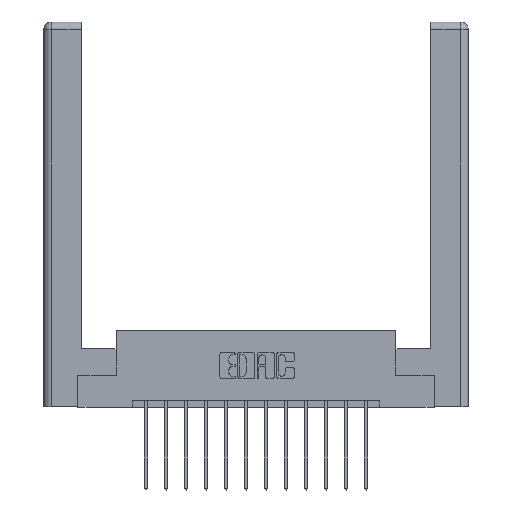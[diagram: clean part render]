
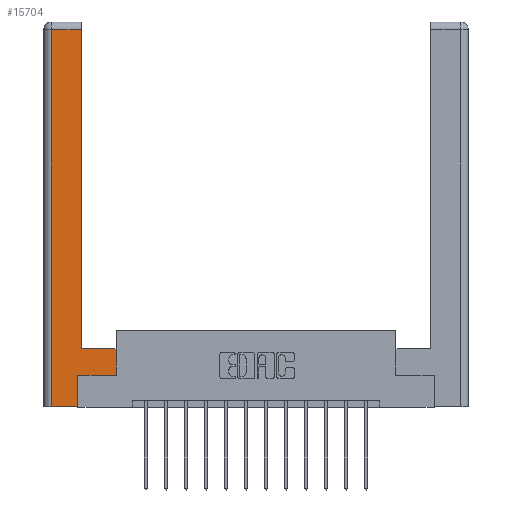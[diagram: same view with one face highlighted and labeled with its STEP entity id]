
A CAD part, top view. The second image highlights one B-rep face of the part: STEP entity #15704.
In plain terms, the highlighted planar face has unit normal (0, 0, 1).
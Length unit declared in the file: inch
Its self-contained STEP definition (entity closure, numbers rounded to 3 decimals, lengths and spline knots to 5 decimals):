
#34 = LINE ( 'NONE', #11506, #3421 ) ;
#152 = EDGE_CURVE ( 'NONE', #5660, #15445, #3620, .T. ) ;
#252 = VERTEX_POINT ( 'NONE', #13423 ) ;
#320 = CARTESIAN_POINT ( 'NONE',  ( 0.265, 0.245, 0. ) ) ;
#393 = CARTESIAN_POINT ( 'NONE',  ( 0.265, 0., 0. ) ) ;
#1141 = FACE_OUTER_BOUND ( 'NONE', #15610, .T. ) ;
#2104 = LINE ( 'NONE', #10669, #11494 ) ;
#2165 = LINE ( 'NONE', #12071, #10993 ) ;
#2635 = VERTEX_POINT ( 'NONE', #12365 ) ;
#2739 = CARTESIAN_POINT ( 'NONE',  ( 0.565, 0.45, 0. ) ) ;
#3310 = DIRECTION ( 'NONE',  ( -1., 0., 0. ) ) ;
#3421 = VECTOR ( 'NONE', #7857, 39.37008 ) ;
#3486 = ORIENTED_EDGE ( 'NONE', *, *, #6939, .T. ) ;
#3620 = LINE ( 'NONE', #11770, #6904 ) ;
#3713 = CARTESIAN_POINT ( 'NONE',  ( 0.0615, 0., 0. ) ) ;
#3792 = ORIENTED_EDGE ( 'NONE', *, *, #14293, .T. ) ;
#3979 = LINE ( 'NONE', #14319, #15554 ) ;
#4308 = ORIENTED_EDGE ( 'NONE', *, *, #7170, .T. ) ;
#4448 = LINE ( 'NONE', #320, #5607 ) ;
#4480 = DIRECTION ( 'NONE',  ( -1., 0., 0. ) ) ;
#4571 = DIRECTION ( 'NONE',  ( 0., 1., 0. ) ) ;
#4984 = CARTESIAN_POINT ( 'NONE',  ( 0.265, 0.245, 0. ) ) ;
#5185 = ORIENTED_EDGE ( 'NONE', *, *, #152, .T. ) ;
#5607 = VECTOR ( 'NONE', #4571, 39.37008 ) ;
#5660 = VERTEX_POINT ( 'NONE', #4984 ) ;
#6153 = VECTOR ( 'NONE', #13874, 39.37008 ) ;
#6904 = VECTOR ( 'NONE', #9497, 39.37008 ) ;
#6939 = EDGE_CURVE ( 'NONE', #7324, #252, #2165, .T. ) ;
#7100 = ORIENTED_EDGE ( 'NONE', *, *, #7383, .T. ) ;
#7170 = EDGE_CURVE ( 'NONE', #2635, #5660, #4448, .T. ) ;
#7324 = VERTEX_POINT ( 'NONE', #9825 ) ;
#7352 = VECTOR ( 'NONE', #12572, 39.37008 ) ;
#7383 = EDGE_CURVE ( 'NONE', #15445, #14016, #15800, .T. ) ;
#7563 = VERTEX_POINT ( 'NONE', #3713 ) ;
#7857 = DIRECTION ( 'NONE',  ( 0., -1., 0. ) ) ;
#8174 = EDGE_CURVE ( 'NONE', #7563, #2635, #12693, .T. ) ;
#8205 = CARTESIAN_POINT ( 'NONE',  ( 0.0615, 2.94, 0. ) ) ;
#8417 = DIRECTION ( 'NONE',  ( 0., 0., -1. ) ) ;
#9130 = EDGE_CURVE ( 'NONE', #14016, #7324, #3979, .T. ) ;
#9189 = EDGE_CURVE ( 'NONE', #252, #15687, #2104, .T. ) ;
#9497 = DIRECTION ( 'NONE',  ( 1., 0., 0. ) ) ;
#9625 = DIRECTION ( 'NONE',  ( -1., 0., 0. ) ) ;
#9825 = CARTESIAN_POINT ( 'NONE',  ( 0.295, 0.45, 0. ) ) ;
#9976 = ORIENTED_EDGE ( 'NONE', *, *, #9189, .T. ) ;
#10096 = CARTESIAN_POINT ( 'NONE',  ( 0.565, 0.45, 0. ) ) ;
#10669 = CARTESIAN_POINT ( 'NONE',  ( 0.0615, 2.94, 0. ) ) ;
#10993 = VECTOR ( 'NONE', #11136, 39.37008 ) ;
#11136 = DIRECTION ( 'NONE',  ( 0., 1., 0. ) ) ;
#11494 = VECTOR ( 'NONE', #3310, 39.37008 ) ;
#11506 = CARTESIAN_POINT ( 'NONE',  ( 0.0615, 0., 0. ) ) ;
#11770 = CARTESIAN_POINT ( 'NONE',  ( 0.565, 0.245, 0. ) ) ;
#12071 = CARTESIAN_POINT ( 'NONE',  ( 0.295, 3., 0. ) ) ;
#12179 = PLANE ( 'NONE',  #12549 ) ;
#12365 = CARTESIAN_POINT ( 'NONE',  ( 0.265, 0., 0. ) ) ;
#12549 = AXIS2_PLACEMENT_3D ( 'NONE', #14591, #8417, #9625 ) ;
#12572 = DIRECTION ( 'NONE',  ( 0., 1., 0. ) ) ;
#12693 = LINE ( 'NONE', #393, #6153 ) ;
#12731 = ORIENTED_EDGE ( 'NONE', *, *, #8174, .T. ) ;
#13423 = CARTESIAN_POINT ( 'NONE',  ( 0.295, 2.94, 0. ) ) ;
#13874 = DIRECTION ( 'NONE',  ( 1., 0., 0. ) ) ;
#14016 = VERTEX_POINT ( 'NONE', #10096 ) ;
#14293 = EDGE_CURVE ( 'NONE', #15687, #7563, #34, .T. ) ;
#14319 = CARTESIAN_POINT ( 'NONE',  ( 0.295, 0.45, 0. ) ) ;
#14569 = ORIENTED_EDGE ( 'NONE', *, *, #9130, .T. ) ;
#14591 = CARTESIAN_POINT ( 'NONE',  ( 0., 0., 0. ) ) ;
#14765 = CARTESIAN_POINT ( 'NONE',  ( 0.565, 0.245, 0. ) ) ;
#15445 = VERTEX_POINT ( 'NONE', #14765 ) ;
#15554 = VECTOR ( 'NONE', #4480, 39.37008 ) ;
#15610 = EDGE_LOOP ( 'NONE', ( #3486, #9976, #3792, #12731, #4308, #5185, #7100, #14569 ) ) ;
#15687 = VERTEX_POINT ( 'NONE', #8205 ) ;
#15704 = ADVANCED_FACE ( 'NONE', ( #1141 ), #12179, .F. ) ;
#15800 = LINE ( 'NONE', #2739, #7352 ) ;
